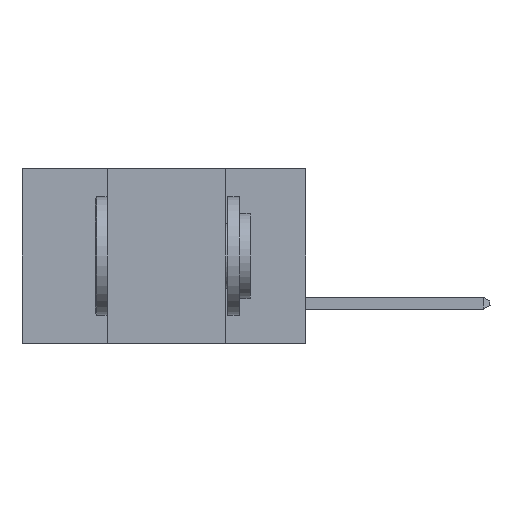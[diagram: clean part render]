
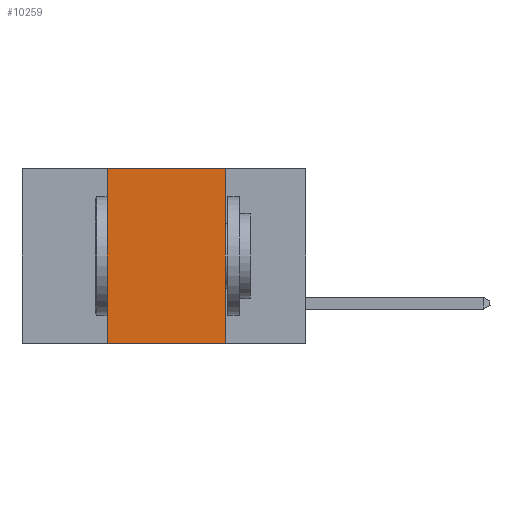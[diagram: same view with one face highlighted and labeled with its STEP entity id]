
A CAD part, left-side view. The second image highlights one B-rep face of the part: STEP entity #10259.
In plain terms, the highlighted planar face has unit normal (-1, 0, 0).
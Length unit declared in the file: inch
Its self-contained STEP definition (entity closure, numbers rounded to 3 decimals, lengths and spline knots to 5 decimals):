
#1159 = DIRECTION ( 'NONE',  ( 1., 0., 0. ) ) ;
#1225 = EDGE_CURVE ( 'NONE', #8683, #25919, #1784, .T. ) ;
#1376 = ORIENTED_EDGE ( 'NONE', *, *, #24131, .F. ) ;
#1586 = CARTESIAN_POINT ( 'NONE',  ( 0., 0.17, -0.37 ) ) ;
#1784 = LINE ( 'NONE', #18288, #8635 ) ;
#1812 = LINE ( 'NONE', #9264, #17807 ) ;
#2059 = VECTOR ( 'NONE', #20042, 39.37008 ) ;
#3718 = AXIS2_PLACEMENT_3D ( 'NONE', #7535, #1159, #9654 ) ;
#5402 = CARTESIAN_POINT ( 'NONE',  ( 0., 0.6, 0. ) ) ;
#6481 = DIRECTION ( 'NONE',  ( 0., -1., 0. ) ) ;
#7535 = CARTESIAN_POINT ( 'NONE',  ( 0., 0.6, 0. ) ) ;
#8247 = LINE ( 'NONE', #12502, #26623 ) ;
#8635 = VECTOR ( 'NONE', #26562, 39.37008 ) ;
#8683 = VERTEX_POINT ( 'NONE', #10227 ) ;
#9260 = VERTEX_POINT ( 'NONE', #1586 ) ;
#9264 = CARTESIAN_POINT ( 'NONE',  ( 0., 0.17, 0. ) ) ;
#9654 = DIRECTION ( 'NONE',  ( 0., 0., -1. ) ) ;
#10227 = CARTESIAN_POINT ( 'NONE',  ( 0., 0.42, -0.37 ) ) ;
#10259 = ADVANCED_FACE ( 'NONE', ( #20313 ), #11728, .F. ) ;
#10822 = EDGE_LOOP ( 'NONE', ( #1376, #14724, #15656, #26349 ) ) ;
#10941 = CARTESIAN_POINT ( 'NONE',  ( 0., 0.17, 0. ) ) ;
#11453 = VERTEX_POINT ( 'NONE', #10941 ) ;
#11728 = PLANE ( 'NONE',  #3718 ) ;
#12502 = CARTESIAN_POINT ( 'NONE',  ( 0., 0.6, -0.37 ) ) ;
#12972 = EDGE_CURVE ( 'NONE', #25919, #11453, #20355, .T. ) ;
#14724 = ORIENTED_EDGE ( 'NONE', *, *, #12972, .F. ) ;
#15296 = CARTESIAN_POINT ( 'NONE',  ( 0., 0.42, 0. ) ) ;
#15656 = ORIENTED_EDGE ( 'NONE', *, *, #1225, .F. ) ;
#17807 = VECTOR ( 'NONE', #23896, 39.37008 ) ;
#18288 = CARTESIAN_POINT ( 'NONE',  ( 0., 0.42, 0. ) ) ;
#20042 = DIRECTION ( 'NONE',  ( 0., -1., 0. ) ) ;
#20313 = FACE_OUTER_BOUND ( 'NONE', #10822, .T. ) ;
#20355 = LINE ( 'NONE', #5402, #2059 ) ;
#23896 = DIRECTION ( 'NONE',  ( 0., 0., -1. ) ) ;
#24131 = EDGE_CURVE ( 'NONE', #11453, #9260, #1812, .T. ) ;
#25480 = EDGE_CURVE ( 'NONE', #8683, #9260, #8247, .T. ) ;
#25919 = VERTEX_POINT ( 'NONE', #15296 ) ;
#26349 = ORIENTED_EDGE ( 'NONE', *, *, #25480, .T. ) ;
#26562 = DIRECTION ( 'NONE',  ( 0., 0., 1. ) ) ;
#26623 = VECTOR ( 'NONE', #6481, 39.37008 ) ;
